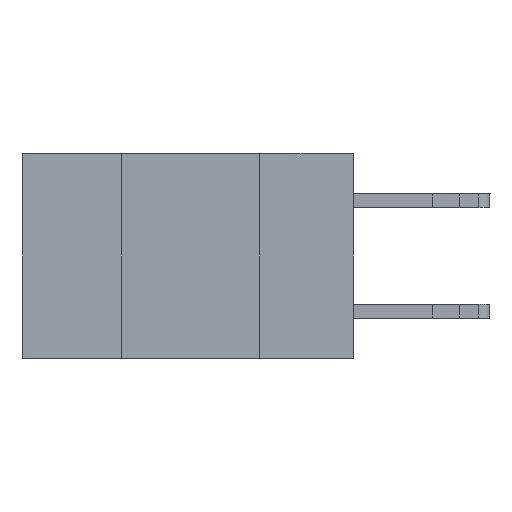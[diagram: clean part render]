
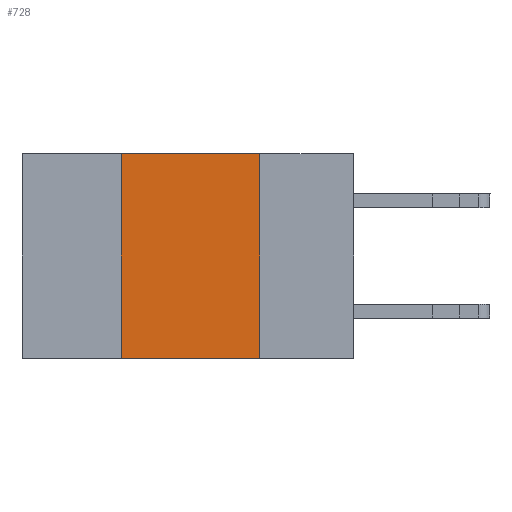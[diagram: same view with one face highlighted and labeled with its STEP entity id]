
A CAD part, left-side view. The second image highlights one B-rep face of the part: STEP entity #728.
In plain terms, the highlighted planar face has unit normal (-1, 0, 0).
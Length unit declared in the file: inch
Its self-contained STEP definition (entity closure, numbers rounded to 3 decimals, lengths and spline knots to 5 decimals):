
#257 = AXIS2_PLACEMENT_3D ( 'NONE', #10903, #17296, #13503 ) ;
#525 = CARTESIAN_POINT ( 'NONE',  ( 0., 0.42, 0. ) ) ;
#728 = ADVANCED_FACE ( 'NONE', ( #4608 ), #17360, .F. ) ;
#998 = DIRECTION ( 'NONE',  ( 0., -1., 0. ) ) ;
#1099 = EDGE_CURVE ( 'NONE', #5821, #20649, #5643, .T. ) ;
#1121 = VECTOR ( 'NONE', #6217, 39.37008 ) ;
#1249 = VECTOR ( 'NONE', #11841, 39.37008 ) ;
#1668 = CARTESIAN_POINT ( 'NONE',  ( 0., 0.17, 0. ) ) ;
#3738 = CARTESIAN_POINT ( 'NONE',  ( 0., 0.17, -0.37 ) ) ;
#4316 = ORIENTED_EDGE ( 'NONE', *, *, #1099, .F. ) ;
#4608 = FACE_OUTER_BOUND ( 'NONE', #9952, .T. ) ;
#4756 = VECTOR ( 'NONE', #12898, 39.37008 ) ;
#5643 = LINE ( 'NONE', #8635, #1121 ) ;
#5821 = VERTEX_POINT ( 'NONE', #8337 ) ;
#6217 = DIRECTION ( 'NONE',  ( 0., 0., 1. ) ) ;
#6322 = CARTESIAN_POINT ( 'NONE',  ( 0., 0.17, 0. ) ) ;
#6561 = ORIENTED_EDGE ( 'NONE', *, *, #9021, .F. ) ;
#7597 = VECTOR ( 'NONE', #998, 39.37008 ) ;
#8337 = CARTESIAN_POINT ( 'NONE',  ( 0., 0.42, -0.37 ) ) ;
#8635 = CARTESIAN_POINT ( 'NONE',  ( 0., 0.42, 0. ) ) ;
#9021 = EDGE_CURVE ( 'NONE', #11281, #13332, #17346, .T. ) ;
#9952 = EDGE_LOOP ( 'NONE', ( #6561, #15780, #4316, #17304 ) ) ;
#10869 = EDGE_CURVE ( 'NONE', #20649, #11281, #20551, .T. ) ;
#10903 = CARTESIAN_POINT ( 'NONE',  ( 0., 0.6, 0. ) ) ;
#11281 = VERTEX_POINT ( 'NONE', #1668 ) ;
#11841 = DIRECTION ( 'NONE',  ( 0., -1., 0. ) ) ;
#12706 = CARTESIAN_POINT ( 'NONE',  ( 0., 0.6, 0. ) ) ;
#12898 = DIRECTION ( 'NONE',  ( 0., 0., -1. ) ) ;
#13332 = VERTEX_POINT ( 'NONE', #3738 ) ;
#13503 = DIRECTION ( 'NONE',  ( 0., 0., -1. ) ) ;
#14870 = EDGE_CURVE ( 'NONE', #5821, #13332, #18835, .T. ) ;
#15780 = ORIENTED_EDGE ( 'NONE', *, *, #10869, .F. ) ;
#17296 = DIRECTION ( 'NONE',  ( 1., 0., 0. ) ) ;
#17304 = ORIENTED_EDGE ( 'NONE', *, *, #14870, .T. ) ;
#17346 = LINE ( 'NONE', #6322, #4756 ) ;
#17360 = PLANE ( 'NONE',  #257 ) ;
#18835 = LINE ( 'NONE', #19877, #1249 ) ;
#19877 = CARTESIAN_POINT ( 'NONE',  ( 0., 0.6, -0.37 ) ) ;
#20551 = LINE ( 'NONE', #12706, #7597 ) ;
#20649 = VERTEX_POINT ( 'NONE', #525 ) ;
